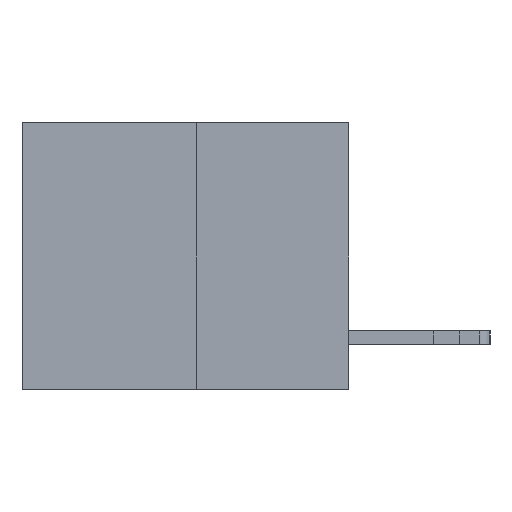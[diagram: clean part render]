
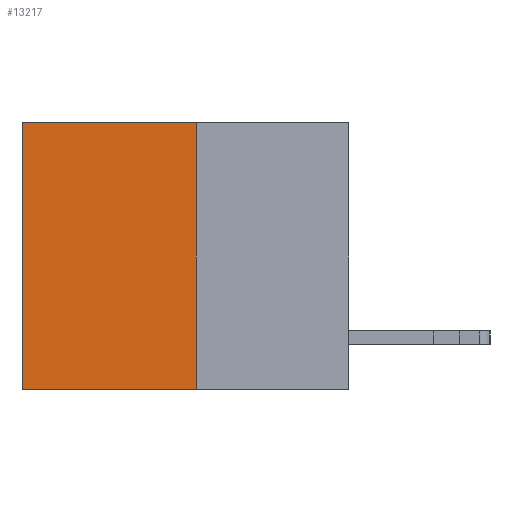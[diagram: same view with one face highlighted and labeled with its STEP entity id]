
A CAD part, left-side view. The second image highlights one B-rep face of the part: STEP entity #13217.
In plain terms, the highlighted planar face has unit normal (-1, 0, 0).
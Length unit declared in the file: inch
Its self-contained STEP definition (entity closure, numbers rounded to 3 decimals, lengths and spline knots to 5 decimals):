
#75 = AXIS2_PLACEMENT_3D ( 'NONE', #23574, #21195, #17115 ) ;
#1386 = EDGE_CURVE ( 'NONE', #20986, #1571, #20793, .T. ) ;
#1571 = VERTEX_POINT ( 'NONE', #26250 ) ;
#3103 = VECTOR ( 'NONE', #6692, 39.37008 ) ;
#4799 = VERTEX_POINT ( 'NONE', #24013 ) ;
#5085 = EDGE_CURVE ( 'NONE', #4799, #14477, #24196, .T. ) ;
#5147 = FACE_OUTER_BOUND ( 'NONE', #14015, .T. ) ;
#5723 = VECTOR ( 'NONE', #11730, 39.37008 ) ;
#5725 = LINE ( 'NONE', #17274, #3103 ) ;
#6692 = DIRECTION ( 'NONE',  ( 0., 0., -1. ) ) ;
#8091 = CARTESIAN_POINT ( 'NONE',  ( 0.3165, 0.28, -0.49 ) ) ;
#8889 = EDGE_CURVE ( 'NONE', #20986, #4799, #5725, .T. ) ;
#11730 = DIRECTION ( 'NONE',  ( 0., 0., -1. ) ) ;
#12534 = ORIENTED_EDGE ( 'NONE', *, *, #8889, .F. ) ;
#13217 = ADVANCED_FACE ( 'NONE', ( #5147 ), #14922, .F. ) ;
#14015 = EDGE_LOOP ( 'NONE', ( #20322, #25481, #12534, #17634 ) ) ;
#14477 = VERTEX_POINT ( 'NONE', #25497 ) ;
#14922 = PLANE ( 'NONE',  #75 ) ;
#16700 = CARTESIAN_POINT ( 'NONE',  ( 0.3165, 0.28, 0. ) ) ;
#17115 = DIRECTION ( 'NONE',  ( 0., 0., -1. ) ) ;
#17239 = VECTOR ( 'NONE', #22975, 39.37008 ) ;
#17274 = CARTESIAN_POINT ( 'NONE',  ( 0.3165, 0.28, -0.49 ) ) ;
#17634 = ORIENTED_EDGE ( 'NONE', *, *, #1386, .T. ) ;
#18437 = DIRECTION ( 'NONE',  ( 0., 1., 0. ) ) ;
#18646 = VECTOR ( 'NONE', #18437, 39.37008 ) ;
#18800 = LINE ( 'NONE', #21940, #5723 ) ;
#20107 = EDGE_CURVE ( 'NONE', #1571, #14477, #18800, .T. ) ;
#20322 = ORIENTED_EDGE ( 'NONE', *, *, #20107, .T. ) ;
#20778 = CARTESIAN_POINT ( 'NONE',  ( 0.3165, 0.28, 0. ) ) ;
#20793 = LINE ( 'NONE', #16700, #17239 ) ;
#20986 = VERTEX_POINT ( 'NONE', #20778 ) ;
#21195 = DIRECTION ( 'NONE',  ( 1., 0., 0. ) ) ;
#21940 = CARTESIAN_POINT ( 'NONE',  ( 0.3165, 0.6, -0.49 ) ) ;
#22975 = DIRECTION ( 'NONE',  ( 0., 1., 0. ) ) ;
#23574 = CARTESIAN_POINT ( 'NONE',  ( 0.3165, 0.28, -0.49 ) ) ;
#24013 = CARTESIAN_POINT ( 'NONE',  ( 0.3165, 0.28, -0.49 ) ) ;
#24196 = LINE ( 'NONE', #8091, #18646 ) ;
#25481 = ORIENTED_EDGE ( 'NONE', *, *, #5085, .F. ) ;
#25497 = CARTESIAN_POINT ( 'NONE',  ( 0.3165, 0.6, -0.49 ) ) ;
#26250 = CARTESIAN_POINT ( 'NONE',  ( 0.3165, 0.6, 0. ) ) ;
